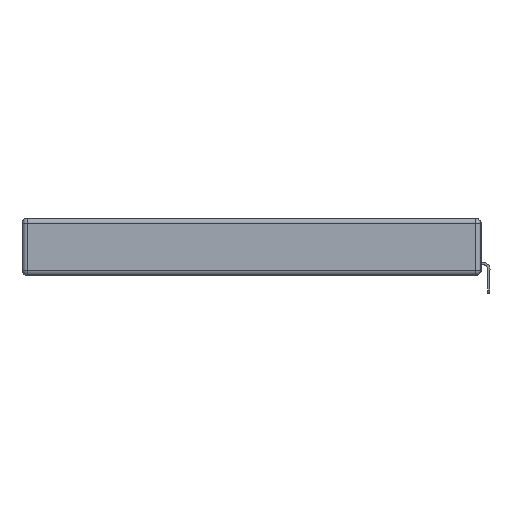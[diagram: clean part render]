
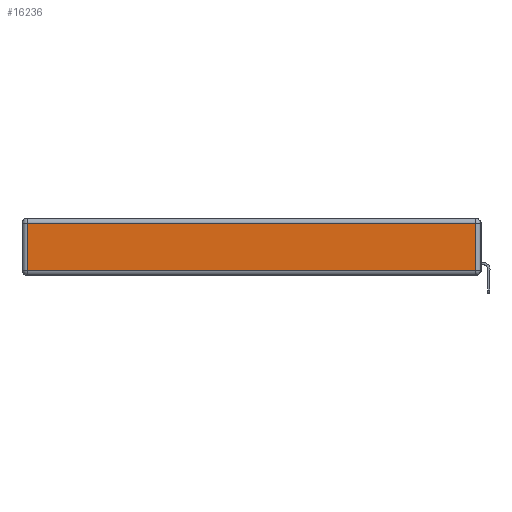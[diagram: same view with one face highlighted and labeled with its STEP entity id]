
A CAD part, left-side view. The second image highlights one B-rep face of the part: STEP entity #16236.
In plain terms, the highlighted planar face has unit normal (-1, 0, 0).
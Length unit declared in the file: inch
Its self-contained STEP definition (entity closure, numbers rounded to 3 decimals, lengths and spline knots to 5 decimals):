
#1114 = LINE ( 'NONE', #8569, #18076 ) ;
#1310 = ORIENTED_EDGE ( 'NONE', *, *, #13361, .T. ) ;
#1635 = VERTEX_POINT ( 'NONE', #2710 ) ;
#2233 = DIRECTION ( 'NONE',  ( 0., -1., 0. ) ) ;
#2411 = VECTOR ( 'NONE', #2446, 39.37008 ) ;
#2446 = DIRECTION ( 'NONE',  ( 0., 1., 0. ) ) ;
#2710 = CARTESIAN_POINT ( 'NONE',  ( 0., 2.72, -0.03 ) ) ;
#3468 = EDGE_CURVE ( 'NONE', #1635, #11743, #18791, .T. ) ;
#4799 = DIRECTION ( 'NONE',  ( 0., 0., 1. ) ) ;
#4876 = DIRECTION ( 'NONE',  ( 0., 0., 1. ) ) ;
#5175 = ORIENTED_EDGE ( 'NONE', *, *, #18813, .T. ) ;
#5276 = EDGE_LOOP ( 'NONE', ( #1310, #5843, #5175, #6940 ) ) ;
#5843 = ORIENTED_EDGE ( 'NONE', *, *, #12480, .T. ) ;
#6281 = VERTEX_POINT ( 'NONE', #9534 ) ;
#6771 = CARTESIAN_POINT ( 'NONE',  ( 0., 2.72, -0.313 ) ) ;
#6940 = ORIENTED_EDGE ( 'NONE', *, *, #3468, .T. ) ;
#7426 = CARTESIAN_POINT ( 'NONE',  ( 0., 2.75, -0.03 ) ) ;
#8262 = DIRECTION ( 'NONE',  ( 0., 0., -1. ) ) ;
#8569 = CARTESIAN_POINT ( 'NONE',  ( 0., 0., -0.313 ) ) ;
#9534 = CARTESIAN_POINT ( 'NONE',  ( 0., 0.03, -0.313 ) ) ;
#11578 = VERTEX_POINT ( 'NONE', #14408 ) ;
#11743 = VERTEX_POINT ( 'NONE', #6771 ) ;
#12480 = EDGE_CURVE ( 'NONE', #6281, #11578, #15033, .T. ) ;
#13084 = PLANE ( 'NONE',  #14890 ) ;
#13361 = EDGE_CURVE ( 'NONE', #11743, #6281, #1114, .T. ) ;
#14408 = CARTESIAN_POINT ( 'NONE',  ( 0., 0.03, -0.03 ) ) ;
#14890 = AXIS2_PLACEMENT_3D ( 'NONE', #19582, #19716, #4876 ) ;
#15033 = LINE ( 'NONE', #21014, #19399 ) ;
#15220 = VECTOR ( 'NONE', #8262, 39.37008 ) ;
#16236 = ADVANCED_FACE ( 'NONE', ( #20237 ), #13084, .T. ) ;
#18076 = VECTOR ( 'NONE', #2233, 39.37008 ) ;
#18791 = LINE ( 'NONE', #21252, #15220 ) ;
#18813 = EDGE_CURVE ( 'NONE', #11578, #1635, #20407, .T. ) ;
#19399 = VECTOR ( 'NONE', #4799, 39.37008 ) ;
#19582 = CARTESIAN_POINT ( 'NONE',  ( 0., 0., -0.343 ) ) ;
#19716 = DIRECTION ( 'NONE',  ( -1., 0., 0. ) ) ;
#20237 = FACE_OUTER_BOUND ( 'NONE', #5276, .T. ) ;
#20407 = LINE ( 'NONE', #7426, #2411 ) ;
#21014 = CARTESIAN_POINT ( 'NONE',  ( 0., 0.03, -0.343 ) ) ;
#21252 = CARTESIAN_POINT ( 'NONE',  ( 0., 2.72, -0.343 ) ) ;
